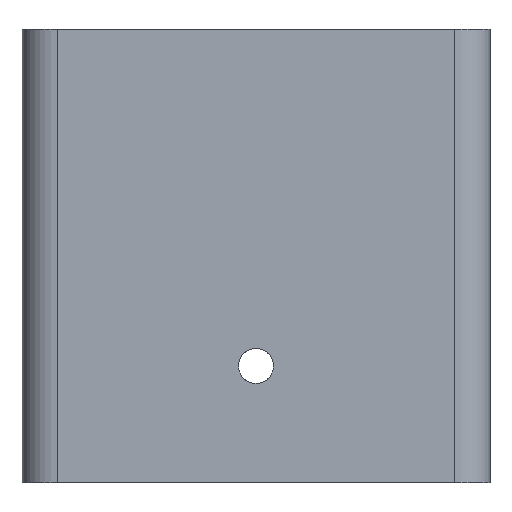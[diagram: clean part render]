
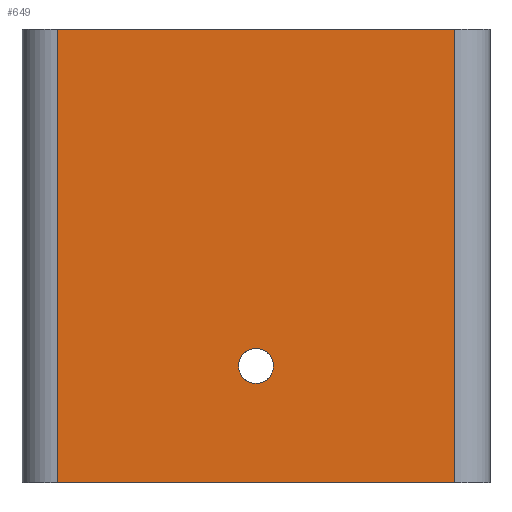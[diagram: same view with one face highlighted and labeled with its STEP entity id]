
A CAD part, front view. The second image highlights one B-rep face of the part: STEP entity #649.
In plain terms, the highlighted planar face has unit normal (0, -1, 0).
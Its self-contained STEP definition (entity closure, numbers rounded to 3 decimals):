
#48=FACE_BOUND('',#122,.T.);
#64=PLANE('',#711);
#80=FACE_OUTER_BOUND('',#121,.T.);
#121=EDGE_LOOP('',(#486,#487,#488,#489));
#122=EDGE_LOOP('',(#490));
#162=LINE('',#915,#212);
#174=LINE('',#954,#224);
#176=LINE('',#958,#226);
#178=LINE('',#973,#228);
#212=VECTOR('',#757,10.);
#224=VECTOR('',#791,10.);
#226=VECTOR('',#795,10.);
#228=VECTOR('',#811,10.);
#276=CIRCLE('',#712,1.5);
#287=VERTEX_POINT('',#912);
#288=VERTEX_POINT('',#914);
#303=VERTEX_POINT('',#950);
#305=VERTEX_POINT('',#957);
#312=VERTEX_POINT('',#974);
#352=EDGE_CURVE('',#287,#288,#162,.T.);
#372=EDGE_CURVE('',#288,#303,#174,.T.);
#374=EDGE_CURVE('',#303,#305,#176,.T.);
#382=EDGE_CURVE('',#305,#287,#178,.T.);
#383=EDGE_CURVE('',#312,#312,#276,.T.);
#486=ORIENTED_EDGE('',*,*,#372,.F.);
#487=ORIENTED_EDGE('',*,*,#352,.F.);
#488=ORIENTED_EDGE('',*,*,#382,.F.);
#489=ORIENTED_EDGE('',*,*,#374,.F.);
#490=ORIENTED_EDGE('',*,*,#383,.T.);
#649=ADVANCED_FACE('',(#80,#48),#64,.F.);
#711=AXIS2_PLACEMENT_3D('',#972,#809,#810);
#712=AXIS2_PLACEMENT_3D('',#975,#812,#813);
#757=DIRECTION('',(1.,0.,0.));
#791=DIRECTION('',(0.,0.,-1.));
#795=DIRECTION('',(-1.,0.,0.));
#809=DIRECTION('center_axis',(0.,1.,0.));
#810=DIRECTION('ref_axis',(0.,0.,-1.));
#811=DIRECTION('',(0.,0.,1.));
#812=DIRECTION('center_axis',(0.,1.,0.));
#813=DIRECTION('ref_axis',(1.,0.,0.));
#912=CARTESIAN_POINT('',(18.,0.,38.8));
#914=CARTESIAN_POINT('',(52.,0.,38.8));
#915=CARTESIAN_POINT('',(35.,0.,38.8));
#950=CARTESIAN_POINT('',(52.,0.,0.));
#954=CARTESIAN_POINT('',(52.,0.,19.4));
#957=CARTESIAN_POINT('',(18.,0.,0.));
#958=CARTESIAN_POINT('',(35.,0.,0.));
#972=CARTESIAN_POINT('Origin',(35.,0.,19.4));
#973=CARTESIAN_POINT('',(18.,0.,19.4));
#974=CARTESIAN_POINT('',(33.5,0.,10.));
#975=CARTESIAN_POINT('Origin',(35.,0.,10.));
